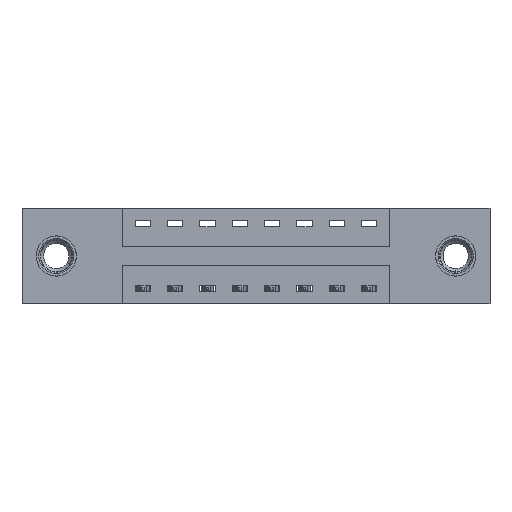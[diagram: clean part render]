
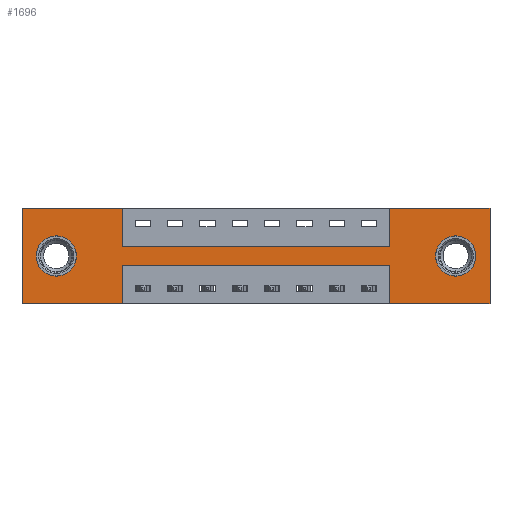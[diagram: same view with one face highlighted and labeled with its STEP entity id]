
A CAD part, front view. The second image highlights one B-rep face of the part: STEP entity #1696.
In plain terms, the highlighted planar face has unit normal (0, -1, 0).
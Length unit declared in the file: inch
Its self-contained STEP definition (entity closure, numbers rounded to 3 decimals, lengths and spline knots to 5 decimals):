
#15 = CARTESIAN_POINT ( 'NONE',  ( 1.4225, 0., -0.37 ) ) ;
#16 = DIRECTION ( 'NONE',  ( 0., 0., 1. ) ) ;
#37 = CARTESIAN_POINT ( 'NONE',  ( 1.4225, 0., 0. ) ) ;
#65 = CARTESIAN_POINT ( 'NONE',  ( 0.3875, 0., -0.15 ) ) ;
#110 = CIRCLE ( 'NONE', #910, 0.078 ) ;
#120 = CARTESIAN_POINT ( 'NONE',  ( 1.4225, 0., -0.15 ) ) ;
#153 = VERTEX_POINT ( 'NONE', #4298 ) ;
#160 = CARTESIAN_POINT ( 'NONE',  ( 0., 0., -0.37 ) ) ;
#179 = VECTOR ( 'NONE', #8352, 39.37008 ) ;
#299 = VERTEX_POINT ( 'NONE', #8614 ) ;
#329 = AXIS2_PLACEMENT_3D ( 'NONE', #9074, #1481, #3291 ) ;
#500 = VERTEX_POINT ( 'NONE', #120 ) ;
#506 = DIRECTION ( 'NONE',  ( -1., 0., 0. ) ) ;
#514 = ORIENTED_EDGE ( 'NONE', *, *, #10150, .F. ) ;
#550 = DIRECTION ( 'NONE',  ( -1., 0., 0. ) ) ;
#601 = EDGE_CURVE ( 'NONE', #3991, #7657, #9660, .T. ) ;
#631 = DIRECTION ( 'NONE',  ( 1., 0., 0. ) ) ;
#673 = DIRECTION ( 'NONE',  ( 0., 0., -1. ) ) ;
#717 = VECTOR ( 'NONE', #8883, 39.37008 ) ;
#721 = ORIENTED_EDGE ( 'NONE', *, *, #601, .F. ) ;
#825 = CARTESIAN_POINT ( 'NONE',  ( 0., 0., 0. ) ) ;
#910 = AXIS2_PLACEMENT_3D ( 'NONE', #4136, #6549, #16 ) ;
#926 = CARTESIAN_POINT ( 'NONE',  ( 0.3875, 0., 0. ) ) ;
#1044 = FACE_BOUND ( 'NONE', #4934, .T. ) ;
#1088 = VECTOR ( 'NONE', #6613, 39.37008 ) ;
#1146 = VERTEX_POINT ( 'NONE', #5130 ) ;
#1154 = CARTESIAN_POINT ( 'NONE',  ( 0.3875, 0., 0. ) ) ;
#1427 = AXIS2_PLACEMENT_3D ( 'NONE', #3242, #1663, #6520 ) ;
#1432 = EDGE_CURVE ( 'NONE', #2604, #10116, #9966, .T. ) ;
#1481 = DIRECTION ( 'NONE',  ( 0., 1., 0. ) ) ;
#1518 = PLANE ( 'NONE',  #6816 ) ;
#1533 = CARTESIAN_POINT ( 'NONE',  ( 1.81, 0., 0. ) ) ;
#1558 = EDGE_CURVE ( 'NONE', #10116, #8213, #7193, .T. ) ;
#1575 = EDGE_CURVE ( 'NONE', #1593, #500, #1744, .T. ) ;
#1593 = VERTEX_POINT ( 'NONE', #10626 ) ;
#1663 = DIRECTION ( 'NONE',  ( 0., 1., 0. ) ) ;
#1696 = ADVANCED_FACE ( 'NONE', ( #1044, #1950, #3219 ), #1518, .T. ) ;
#1744 = LINE ( 'NONE', #65, #6476 ) ;
#1851 = VERTEX_POINT ( 'NONE', #1154 ) ;
#1949 = EDGE_CURVE ( 'NONE', #8213, #4465, #8931, .T. ) ;
#1950 = FACE_BOUND ( 'NONE', #9143, .T. ) ;
#1955 = ORIENTED_EDGE ( 'NONE', *, *, #9836, .F. ) ;
#2032 = CARTESIAN_POINT ( 'NONE',  ( 0.3875, 0., -0.37 ) ) ;
#2343 = CARTESIAN_POINT ( 'NONE',  ( 1.81, 0., -0.37 ) ) ;
#2359 = CIRCLE ( 'NONE', #329, 0.078 ) ;
#2486 = DIRECTION ( 'NONE',  ( 0., -1., 0. ) ) ;
#2604 = VERTEX_POINT ( 'NONE', #2343 ) ;
#2702 = CIRCLE ( 'NONE', #10597, 0.078 ) ;
#2744 = CIRCLE ( 'NONE', #1427, 0.078 ) ;
#2751 = LINE ( 'NONE', #37, #179 ) ;
#2785 = ORIENTED_EDGE ( 'NONE', *, *, #9664, .T. ) ;
#2823 = CARTESIAN_POINT ( 'NONE',  ( 1.6775, 0., -0.107 ) ) ;
#3054 = CARTESIAN_POINT ( 'NONE',  ( 1.6775, 0., -0.185 ) ) ;
#3140 = VECTOR ( 'NONE', #5017, 39.37008 ) ;
#3219 = FACE_OUTER_BOUND ( 'NONE', #3849, .T. ) ;
#3242 = CARTESIAN_POINT ( 'NONE',  ( 1.6775, 0., -0.185 ) ) ;
#3291 = DIRECTION ( 'NONE',  ( 0., 0., 1. ) ) ;
#3402 = ORIENTED_EDGE ( 'NONE', *, *, #1949, .F. ) ;
#3448 = CARTESIAN_POINT ( 'NONE',  ( 1.6775, 0., -0.263 ) ) ;
#3693 = ORIENTED_EDGE ( 'NONE', *, *, #6618, .F. ) ;
#3710 = VECTOR ( 'NONE', #673, 39.37008 ) ;
#3813 = ORIENTED_EDGE ( 'NONE', *, *, #9161, .F. ) ;
#3832 = VECTOR ( 'NONE', #9553, 39.37008 ) ;
#3849 = EDGE_LOOP ( 'NONE', ( #5784, #3402, #6526, #9647, #3693, #514, #1955, #6310, #9944, #3813, #721, #8507 ) ) ;
#3892 = DIRECTION ( 'NONE',  ( 0., 1., 0. ) ) ;
#3991 = VERTEX_POINT ( 'NONE', #160 ) ;
#4136 = CARTESIAN_POINT ( 'NONE',  ( 0.1325, 0., -0.185 ) ) ;
#4298 = CARTESIAN_POINT ( 'NONE',  ( 0.3875, 0., -0.37 ) ) ;
#4350 = DIRECTION ( 'NONE',  ( 0., 0., 1. ) ) ;
#4465 = VERTEX_POINT ( 'NONE', #7562 ) ;
#4728 = CARTESIAN_POINT ( 'NONE',  ( 1.81, 0., 0. ) ) ;
#4934 = EDGE_LOOP ( 'NONE', ( #6264, #9845 ) ) ;
#4969 = ORIENTED_EDGE ( 'NONE', *, *, #7394, .T. ) ;
#4971 = VERTEX_POINT ( 'NONE', #3448 ) ;
#5017 = DIRECTION ( 'NONE',  ( 0., 0., -1. ) ) ;
#5092 = EDGE_CURVE ( 'NONE', #4971, #8313, #2744, .T. ) ;
#5130 = CARTESIAN_POINT ( 'NONE',  ( 0.1325, 0., -0.263 ) ) ;
#5136 = VECTOR ( 'NONE', #5324, 39.37008 ) ;
#5184 = CARTESIAN_POINT ( 'NONE',  ( 0., 0., 0. ) ) ;
#5324 = DIRECTION ( 'NONE',  ( 0., 0., -1. ) ) ;
#5489 = DIRECTION ( 'NONE',  ( 0., 0., -1. ) ) ;
#5782 = DIRECTION ( 'NONE',  ( 1., 0., 0. ) ) ;
#5784 = ORIENTED_EDGE ( 'NONE', *, *, #10574, .F. ) ;
#5835 = VECTOR ( 'NONE', #4350, 39.37008 ) ;
#6167 = VECTOR ( 'NONE', #506, 39.37008 ) ;
#6264 = ORIENTED_EDGE ( 'NONE', *, *, #6657, .T. ) ;
#6310 = ORIENTED_EDGE ( 'NONE', *, *, #1575, .F. ) ;
#6476 = VECTOR ( 'NONE', #5782, 39.37008 ) ;
#6520 = DIRECTION ( 'NONE',  ( 0., 0., -1. ) ) ;
#6526 = ORIENTED_EDGE ( 'NONE', *, *, #1558, .F. ) ;
#6549 = DIRECTION ( 'NONE',  ( 0., 1., 0. ) ) ;
#6613 = DIRECTION ( 'NONE',  ( 1., 0., 0. ) ) ;
#6618 = EDGE_CURVE ( 'NONE', #10322, #2604, #7466, .T. ) ;
#6657 = EDGE_CURVE ( 'NONE', #8313, #4971, #2702, .T. ) ;
#6816 = AXIS2_PLACEMENT_3D ( 'NONE', #9120, #2486, #7317 ) ;
#7034 = CARTESIAN_POINT ( 'NONE',  ( 0., 0., -0.37 ) ) ;
#7193 = LINE ( 'NONE', #15, #717 ) ;
#7317 = DIRECTION ( 'NONE',  ( 0., 0., -1. ) ) ;
#7335 = LINE ( 'NONE', #2032, #5136 ) ;
#7394 = EDGE_CURVE ( 'NONE', #1146, #299, #110, .T. ) ;
#7466 = LINE ( 'NONE', #4728, #3710 ) ;
#7562 = CARTESIAN_POINT ( 'NONE',  ( 0.3875, 0., -0.22 ) ) ;
#7657 = VERTEX_POINT ( 'NONE', #5184 ) ;
#7708 = LINE ( 'NONE', #926, #3140 ) ;
#7883 = LINE ( 'NONE', #7034, #3832 ) ;
#7935 = LINE ( 'NONE', #9779, #8958 ) ;
#7994 = CARTESIAN_POINT ( 'NONE',  ( 0.3875, 0., -0.22 ) ) ;
#8105 = CARTESIAN_POINT ( 'NONE',  ( 1.4225, 0., 0. ) ) ;
#8116 = VERTEX_POINT ( 'NONE', #8105 ) ;
#8213 = VERTEX_POINT ( 'NONE', #8403 ) ;
#8313 = VERTEX_POINT ( 'NONE', #2823 ) ;
#8352 = DIRECTION ( 'NONE',  ( 0., 0., 1. ) ) ;
#8403 = CARTESIAN_POINT ( 'NONE',  ( 1.4225, 0., -0.22 ) ) ;
#8507 = ORIENTED_EDGE ( 'NONE', *, *, #10751, .F. ) ;
#8590 = CARTESIAN_POINT ( 'NONE',  ( 0., 0., 0. ) ) ;
#8614 = CARTESIAN_POINT ( 'NONE',  ( 0.1325, 0., -0.107 ) ) ;
#8712 = EDGE_CURVE ( 'NONE', #1851, #1593, #7708, .T. ) ;
#8743 = LINE ( 'NONE', #825, #1088 ) ;
#8883 = DIRECTION ( 'NONE',  ( 0., 0., 1. ) ) ;
#8931 = LINE ( 'NONE', #7994, #6167 ) ;
#8958 = VECTOR ( 'NONE', #631, 39.37008 ) ;
#9074 = CARTESIAN_POINT ( 'NONE',  ( 0.1325, 0., -0.185 ) ) ;
#9120 = CARTESIAN_POINT ( 'NONE',  ( 0., 0., -0.37 ) ) ;
#9143 = EDGE_LOOP ( 'NONE', ( #2785, #4969 ) ) ;
#9161 = EDGE_CURVE ( 'NONE', #7657, #1851, #8743, .T. ) ;
#9553 = DIRECTION ( 'NONE',  ( -1., 0., 0. ) ) ;
#9647 = ORIENTED_EDGE ( 'NONE', *, *, #1432, .F. ) ;
#9660 = LINE ( 'NONE', #8590, #5835 ) ;
#9664 = EDGE_CURVE ( 'NONE', #299, #1146, #2359, .T. ) ;
#9703 = CARTESIAN_POINT ( 'NONE',  ( 0., 0., -0.37 ) ) ;
#9779 = CARTESIAN_POINT ( 'NONE',  ( 0., 0., 0. ) ) ;
#9811 = VECTOR ( 'NONE', #550, 39.37008 ) ;
#9836 = EDGE_CURVE ( 'NONE', #500, #8116, #2751, .T. ) ;
#9845 = ORIENTED_EDGE ( 'NONE', *, *, #5092, .T. ) ;
#9944 = ORIENTED_EDGE ( 'NONE', *, *, #8712, .F. ) ;
#9966 = LINE ( 'NONE', #9703, #9811 ) ;
#10116 = VERTEX_POINT ( 'NONE', #10394 ) ;
#10150 = EDGE_CURVE ( 'NONE', #8116, #10322, #7935, .T. ) ;
#10322 = VERTEX_POINT ( 'NONE', #1533 ) ;
#10394 = CARTESIAN_POINT ( 'NONE',  ( 1.4225, 0., -0.37 ) ) ;
#10574 = EDGE_CURVE ( 'NONE', #4465, #153, #7335, .T. ) ;
#10597 = AXIS2_PLACEMENT_3D ( 'NONE', #3054, #3892, #5489 ) ;
#10626 = CARTESIAN_POINT ( 'NONE',  ( 0.3875, 0., -0.15 ) ) ;
#10751 = EDGE_CURVE ( 'NONE', #153, #3991, #7883, .T. ) ;
